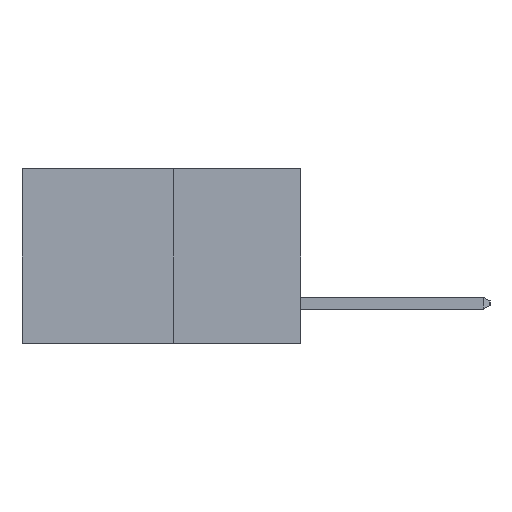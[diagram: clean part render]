
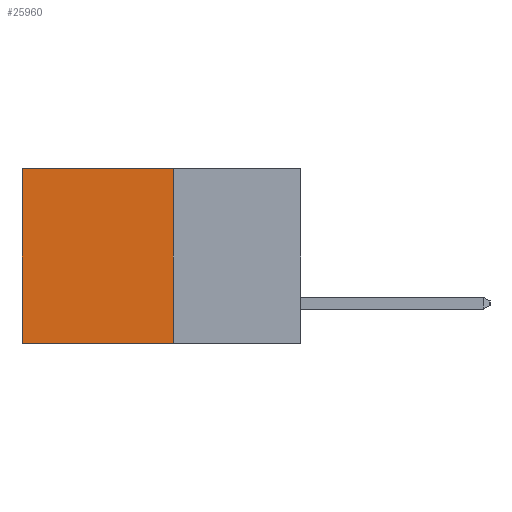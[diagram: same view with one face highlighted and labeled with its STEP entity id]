
A CAD part, left-side view. The second image highlights one B-rep face of the part: STEP entity #25960.
In plain terms, the highlighted planar face has unit normal (-1, 0, 0).
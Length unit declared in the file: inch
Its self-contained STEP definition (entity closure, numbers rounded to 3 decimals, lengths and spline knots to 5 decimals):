
#1090 = CARTESIAN_POINT ( 'NONE',  ( 0.277, 0.27, 0. ) ) ;
#2087 = DIRECTION ( 'NONE',  ( 0., 0., -1. ) ) ;
#3198 = CARTESIAN_POINT ( 'NONE',  ( 0.277, 0.27, -0.37 ) ) ;
#3201 = CARTESIAN_POINT ( 'NONE',  ( 0.277, 0.59, -0.37 ) ) ;
#3818 = ORIENTED_EDGE ( 'NONE', *, *, #29035, .F. ) ;
#4589 = LINE ( 'NONE', #19477, #28088 ) ;
#4624 = CARTESIAN_POINT ( 'NONE',  ( 0.277, 0.27, -0.37 ) ) ;
#5335 = ORIENTED_EDGE ( 'NONE', *, *, #10210, .T. ) ;
#6070 = EDGE_CURVE ( 'NONE', #6366, #13398, #11160, .T. ) ;
#6172 = VECTOR ( 'NONE', #2087, 39.37008 ) ;
#6311 = DIRECTION ( 'NONE',  ( 0., 0., -1. ) ) ;
#6366 = VERTEX_POINT ( 'NONE', #25491 ) ;
#7362 = ORIENTED_EDGE ( 'NONE', *, *, #6070, .T. ) ;
#7591 = CARTESIAN_POINT ( 'NONE',  ( 0.277, 0.27, -0.37 ) ) ;
#7683 = DIRECTION ( 'NONE',  ( 0., 0., -1. ) ) ;
#8147 = VECTOR ( 'NONE', #25158, 39.37008 ) ;
#8859 = LINE ( 'NONE', #4624, #8147 ) ;
#9521 = VERTEX_POINT ( 'NONE', #1090 ) ;
#10210 = EDGE_CURVE ( 'NONE', #9521, #6366, #4589, .T. ) ;
#11160 = LINE ( 'NONE', #17621, #17134 ) ;
#13253 = EDGE_LOOP ( 'NONE', ( #7362, #15764, #3818, #5335 ) ) ;
#13398 = VERTEX_POINT ( 'NONE', #3201 ) ;
#14621 = EDGE_CURVE ( 'NONE', #23745, #13398, #8859, .T. ) ;
#15764 = ORIENTED_EDGE ( 'NONE', *, *, #14621, .F. ) ;
#16082 = AXIS2_PLACEMENT_3D ( 'NONE', #7591, #21254, #7683 ) ;
#17134 = VECTOR ( 'NONE', #6311, 39.37008 ) ;
#17621 = CARTESIAN_POINT ( 'NONE',  ( 0.277, 0.59, -0.37 ) ) ;
#18288 = LINE ( 'NONE', #29421, #6172 ) ;
#18993 = PLANE ( 'NONE',  #16082 ) ;
#19477 = CARTESIAN_POINT ( 'NONE',  ( 0.277, 0.27, 0. ) ) ;
#19657 = FACE_OUTER_BOUND ( 'NONE', #13253, .T. ) ;
#21254 = DIRECTION ( 'NONE',  ( 1., 0., 0. ) ) ;
#21724 = DIRECTION ( 'NONE',  ( 0., 1., 0. ) ) ;
#23745 = VERTEX_POINT ( 'NONE', #3198 ) ;
#25158 = DIRECTION ( 'NONE',  ( 0., 1., 0. ) ) ;
#25491 = CARTESIAN_POINT ( 'NONE',  ( 0.277, 0.59, 0. ) ) ;
#25960 = ADVANCED_FACE ( 'NONE', ( #19657 ), #18993, .F. ) ;
#28088 = VECTOR ( 'NONE', #21724, 39.37008 ) ;
#29035 = EDGE_CURVE ( 'NONE', #9521, #23745, #18288, .T. ) ;
#29421 = CARTESIAN_POINT ( 'NONE',  ( 0.277, 0.27, -0.37 ) ) ;
